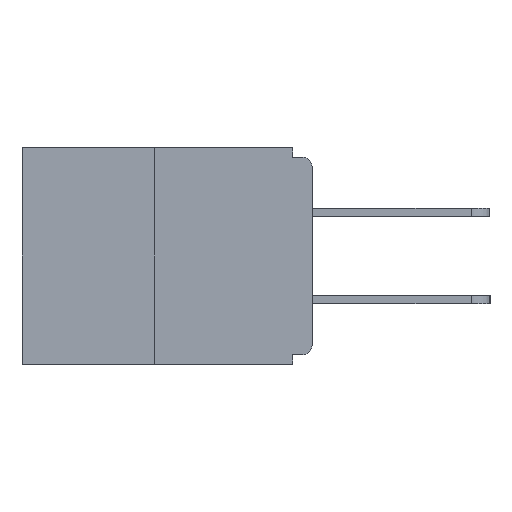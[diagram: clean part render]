
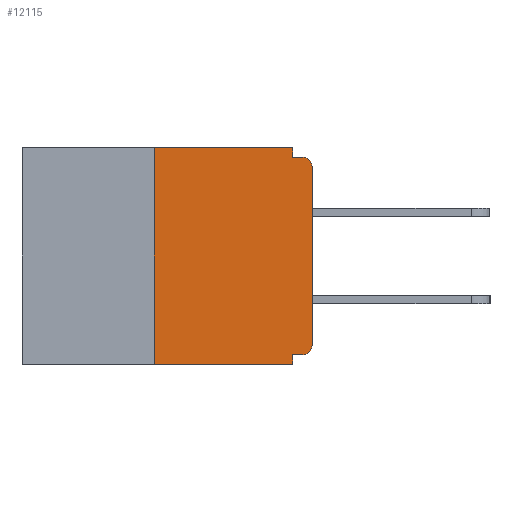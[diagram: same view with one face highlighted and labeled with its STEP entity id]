
A CAD part, left-side view. The second image highlights one B-rep face of the part: STEP entity #12115.
In plain terms, the highlighted planar face has unit normal (-1, 0, 0).
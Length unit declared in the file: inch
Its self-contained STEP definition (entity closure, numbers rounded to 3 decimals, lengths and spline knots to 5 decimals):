
#47 = CARTESIAN_POINT ( 'NONE',  ( 0., 0.031, -0.015 ) ) ;
#185 = CARTESIAN_POINT ( 'NONE',  ( 0., 0.031, 0. ) ) ;
#259 = PLANE ( 'NONE',  #3534 ) ;
#482 = VECTOR ( 'NONE', #12528, 39.37008 ) ;
#610 = ORIENTED_EDGE ( 'NONE', *, *, #12441, .F. ) ;
#611 = DIRECTION ( 'NONE',  ( -1., 0., 0. ) ) ;
#1105 = CARTESIAN_POINT ( 'NONE',  ( 0., 0.25, 0. ) ) ;
#1113 = CARTESIAN_POINT ( 'NONE',  ( 0., 0.25, 0. ) ) ;
#1476 = EDGE_CURVE ( 'NONE', #14167, #13481, #8209, .T. ) ;
#1508 = AXIS2_PLACEMENT_3D ( 'NONE', #4056, #611, #12044 ) ;
#1532 = ORIENTED_EDGE ( 'NONE', *, *, #6999, .F. ) ;
#1853 = CARTESIAN_POINT ( 'NONE',  ( 0., 0.46, 0. ) ) ;
#1992 = ORIENTED_EDGE ( 'NONE', *, *, #1476, .F. ) ;
#2019 = CIRCLE ( 'NONE', #1508, 0.015 ) ;
#2119 = ORIENTED_EDGE ( 'NONE', *, *, #7200, .F. ) ;
#2462 = ORIENTED_EDGE ( 'NONE', *, *, #3986, .F. ) ;
#2640 = CARTESIAN_POINT ( 'NONE',  ( 0., 0.031, -0.343 ) ) ;
#2674 = VERTEX_POINT ( 'NONE', #47 ) ;
#2675 = CARTESIAN_POINT ( 'NONE',  ( 0., 0.015, -0.015 ) ) ;
#3133 = LINE ( 'NONE', #3195, #9857 ) ;
#3195 = CARTESIAN_POINT ( 'NONE',  ( 0., 0., 0. ) ) ;
#3315 = DIRECTION ( 'NONE',  ( 0., 0., 1. ) ) ;
#3534 = AXIS2_PLACEMENT_3D ( 'NONE', #5986, #10399, #3635 ) ;
#3548 = LINE ( 'NONE', #9108, #12952 ) ;
#3635 = DIRECTION ( 'NONE',  ( 0., 0., -1. ) ) ;
#3687 = EDGE_CURVE ( 'NONE', #7178, #13481, #12864, .T. ) ;
#3986 = EDGE_CURVE ( 'NONE', #8582, #14167, #14643, .T. ) ;
#4056 = CARTESIAN_POINT ( 'NONE',  ( 0., 0.015, -0.03 ) ) ;
#4248 = LINE ( 'NONE', #4583, #482 ) ;
#4321 = DIRECTION ( 'NONE',  ( 0., 0., 1. ) ) ;
#4583 = CARTESIAN_POINT ( 'NONE',  ( 0., 0., -0.015 ) ) ;
#4683 = VECTOR ( 'NONE', #10553, 39.37008 ) ;
#4735 = ORIENTED_EDGE ( 'NONE', *, *, #8794, .T. ) ;
#4810 = DIRECTION ( 'NONE',  ( 0., 0., -1. ) ) ;
#5311 = VECTOR ( 'NONE', #3315, 39.37008 ) ;
#5333 = DIRECTION ( 'NONE',  ( 0., 1., 0. ) ) ;
#5956 = VERTEX_POINT ( 'NONE', #1113 ) ;
#5969 = LINE ( 'NONE', #1853, #11476 ) ;
#5986 = CARTESIAN_POINT ( 'NONE',  ( 0., 0.46, 0. ) ) ;
#6208 = ORIENTED_EDGE ( 'NONE', *, *, #3687, .T. ) ;
#6649 = CARTESIAN_POINT ( 'NONE',  ( 0., 0.46, -0.343 ) ) ;
#6999 = EDGE_CURVE ( 'NONE', #11519, #2674, #3548, .T. ) ;
#7178 = VERTEX_POINT ( 'NONE', #11474 ) ;
#7200 = EDGE_CURVE ( 'NONE', #2674, #10295, #4248, .T. ) ;
#7608 = CARTESIAN_POINT ( 'NONE',  ( 0., 0., -0.328 ) ) ;
#8020 = DIRECTION ( 'NONE',  ( -1., 0., 0. ) ) ;
#8209 = LINE ( 'NONE', #2640, #4683 ) ;
#8491 = VERTEX_POINT ( 'NONE', #11931 ) ;
#8582 = VERTEX_POINT ( 'NONE', #13005 ) ;
#8720 = CARTESIAN_POINT ( 'NONE',  ( 0., 0., -0.313 ) ) ;
#8794 = EDGE_CURVE ( 'NONE', #9949, #8491, #3133, .T. ) ;
#9108 = CARTESIAN_POINT ( 'NONE',  ( 0., 0.031, 0. ) ) ;
#9152 = EDGE_CURVE ( 'NONE', #8491, #10295, #2019, .T. ) ;
#9857 = VECTOR ( 'NONE', #4321, 39.37008 ) ;
#9904 = CARTESIAN_POINT ( 'NONE',  ( 0., 0.031, -0.343 ) ) ;
#9949 = VERTEX_POINT ( 'NONE', #8720 ) ;
#9970 = DIRECTION ( 'NONE',  ( 0., -1., 0. ) ) ;
#10295 = VERTEX_POINT ( 'NONE', #2675 ) ;
#10348 = VECTOR ( 'NONE', #14593, 39.37008 ) ;
#10399 = DIRECTION ( 'NONE',  ( 1., 0., 0. ) ) ;
#10553 = DIRECTION ( 'NONE',  ( 0., 0., -1. ) ) ;
#10646 = FACE_OUTER_BOUND ( 'NONE', #13026, .T. ) ;
#11253 = ORIENTED_EDGE ( 'NONE', *, *, #11534, .T. ) ;
#11339 = LINE ( 'NONE', #1105, #5311 ) ;
#11474 = CARTESIAN_POINT ( 'NONE',  ( 0., 0.25, -0.343 ) ) ;
#11476 = VECTOR ( 'NONE', #9970, 39.37008 ) ;
#11519 = VERTEX_POINT ( 'NONE', #185 ) ;
#11534 = EDGE_CURVE ( 'NONE', #8582, #9949, #12646, .T. ) ;
#11784 = AXIS2_PLACEMENT_3D ( 'NONE', #12614, #8020, #4810 ) ;
#11931 = CARTESIAN_POINT ( 'NONE',  ( 0., 0., -0.03 ) ) ;
#12044 = DIRECTION ( 'NONE',  ( 0., 0., -1. ) ) ;
#12115 = ADVANCED_FACE ( 'NONE', ( #10646 ), #259, .F. ) ;
#12314 = VECTOR ( 'NONE', #5333, 39.37008 ) ;
#12408 = ORIENTED_EDGE ( 'NONE', *, *, #14721, .F. ) ;
#12441 = EDGE_CURVE ( 'NONE', #7178, #5956, #11339, .T. ) ;
#12528 = DIRECTION ( 'NONE',  ( 0., -1., 0. ) ) ;
#12614 = CARTESIAN_POINT ( 'NONE',  ( 0., 0.015, -0.313 ) ) ;
#12646 = CIRCLE ( 'NONE', #11784, 0.015 ) ;
#12864 = LINE ( 'NONE', #6649, #10348 ) ;
#12952 = VECTOR ( 'NONE', #13798, 39.37008 ) ;
#13005 = CARTESIAN_POINT ( 'NONE',  ( 0., 0.015, -0.328 ) ) ;
#13026 = EDGE_LOOP ( 'NONE', ( #12408, #610, #6208, #1992, #2462, #11253, #4735, #13989, #2119, #1532 ) ) ;
#13481 = VERTEX_POINT ( 'NONE', #9904 ) ;
#13798 = DIRECTION ( 'NONE',  ( 0., 0., -1. ) ) ;
#13989 = ORIENTED_EDGE ( 'NONE', *, *, #9152, .T. ) ;
#14167 = VERTEX_POINT ( 'NONE', #14637 ) ;
#14593 = DIRECTION ( 'NONE',  ( 0., -1., 0. ) ) ;
#14637 = CARTESIAN_POINT ( 'NONE',  ( 0., 0.031, -0.328 ) ) ;
#14643 = LINE ( 'NONE', #7608, #12314 ) ;
#14721 = EDGE_CURVE ( 'NONE', #5956, #11519, #5969, .T. ) ;
